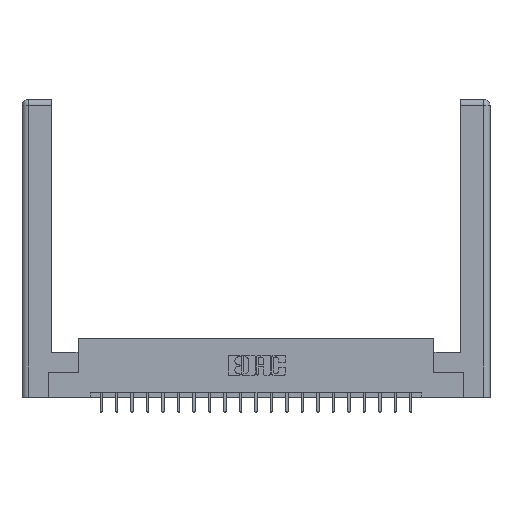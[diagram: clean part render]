
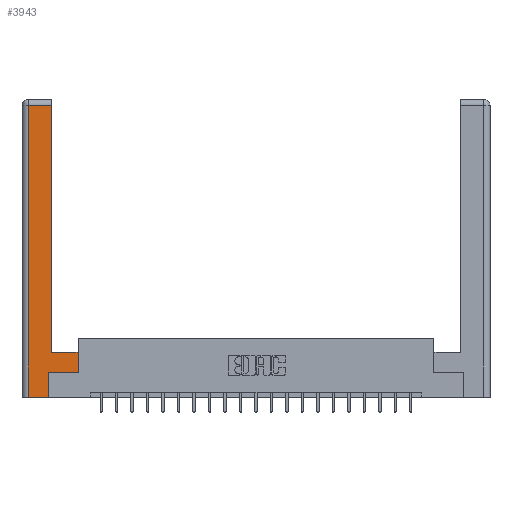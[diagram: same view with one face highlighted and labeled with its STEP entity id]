
A CAD part, top view. The second image highlights one B-rep face of the part: STEP entity #3943.
In plain terms, the highlighted planar face has unit normal (0, 0, 1).
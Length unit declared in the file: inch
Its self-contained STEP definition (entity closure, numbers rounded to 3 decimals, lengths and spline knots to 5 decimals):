
#540 = LINE ( 'NONE', #18890, #16519 ) ;
#795 = DIRECTION ( 'NONE',  ( -1., 0., 0. ) ) ;
#811 = EDGE_LOOP ( 'NONE', ( #6011, #13386, #1071, #17610, #8185, #5318, #9160, #10498 ) ) ;
#840 = VECTOR ( 'NONE', #19273, 39.37008 ) ;
#893 = EDGE_CURVE ( 'NONE', #18559, #1119, #18105, .T. ) ;
#1071 = ORIENTED_EDGE ( 'NONE', *, *, #3435, .T. ) ;
#1119 = VERTEX_POINT ( 'NONE', #12727 ) ;
#1595 = EDGE_CURVE ( 'NONE', #2181, #20528, #540, .T. ) ;
#2181 = VERTEX_POINT ( 'NONE', #11145 ) ;
#2220 = CARTESIAN_POINT ( 'NONE',  ( 0.295, 2.94, 0. ) ) ;
#2565 = EDGE_CURVE ( 'NONE', #6105, #2181, #20928, .T. ) ;
#3435 = EDGE_CURVE ( 'NONE', #1119, #8677, #11996, .T. ) ;
#3753 = CARTESIAN_POINT ( 'NONE',  ( 0.0615, 0., 0. ) ) ;
#3825 = DIRECTION ( 'NONE',  ( -1., 0., 0. ) ) ;
#3943 = ADVANCED_FACE ( 'NONE', ( #18073 ), #9119, .F. ) ;
#5196 = EDGE_CURVE ( 'NONE', #15218, #6105, #16228, .T. ) ;
#5318 = ORIENTED_EDGE ( 'NONE', *, *, #5196, .T. ) ;
#5911 = CARTESIAN_POINT ( 'NONE',  ( 0., 0., 0. ) ) ;
#6011 = ORIENTED_EDGE ( 'NONE', *, *, #12866, .T. ) ;
#6105 = VERTEX_POINT ( 'NONE', #11864 ) ;
#7302 = CARTESIAN_POINT ( 'NONE',  ( 0.0615, 2.94, 0. ) ) ;
#7859 = VECTOR ( 'NONE', #21332, 39.37008 ) ;
#7906 = VERTEX_POINT ( 'NONE', #12146 ) ;
#7962 = EDGE_CURVE ( 'NONE', #7906, #15218, #21311, .T. ) ;
#8045 = VECTOR ( 'NONE', #16902, 39.37008 ) ;
#8185 = ORIENTED_EDGE ( 'NONE', *, *, #7962, .T. ) ;
#8485 = CARTESIAN_POINT ( 'NONE',  ( 0.565, 0.45, 0. ) ) ;
#8677 = VERTEX_POINT ( 'NONE', #3753 ) ;
#9119 = PLANE ( 'NONE',  #15578 ) ;
#9160 = ORIENTED_EDGE ( 'NONE', *, *, #2565, .T. ) ;
#9291 = EDGE_CURVE ( 'NONE', #8677, #7906, #17596, .T. ) ;
#9335 = CARTESIAN_POINT ( 'NONE',  ( 0.295, 0.45, 0. ) ) ;
#9448 = CARTESIAN_POINT ( 'NONE',  ( 0.265, 0., 0. ) ) ;
#10498 = ORIENTED_EDGE ( 'NONE', *, *, #1595, .T. ) ;
#10689 = DIRECTION ( 'NONE',  ( 0., 1., 0. ) ) ;
#10810 = DIRECTION ( 'NONE',  ( -1., 0., 0. ) ) ;
#11069 = DIRECTION ( 'NONE',  ( 1., 0., 0. ) ) ;
#11145 = CARTESIAN_POINT ( 'NONE',  ( 0.565, 0.45, 0. ) ) ;
#11864 = CARTESIAN_POINT ( 'NONE',  ( 0.565, 0.245, 0. ) ) ;
#11996 = LINE ( 'NONE', #15237, #8045 ) ;
#12146 = CARTESIAN_POINT ( 'NONE',  ( 0.265, 0., 0. ) ) ;
#12727 = CARTESIAN_POINT ( 'NONE',  ( 0.0615, 2.94, 0. ) ) ;
#12866 = EDGE_CURVE ( 'NONE', #20528, #18559, #19707, .T. ) ;
#13386 = ORIENTED_EDGE ( 'NONE', *, *, #893, .T. ) ;
#14033 = CARTESIAN_POINT ( 'NONE',  ( 0.295, 3., 0. ) ) ;
#15218 = VERTEX_POINT ( 'NONE', #21317 ) ;
#15237 = CARTESIAN_POINT ( 'NONE',  ( 0.0615, 0., 0. ) ) ;
#15578 = AXIS2_PLACEMENT_3D ( 'NONE', #5911, #15795, #10810 ) ;
#15795 = DIRECTION ( 'NONE',  ( 0., 0., -1. ) ) ;
#16105 = CARTESIAN_POINT ( 'NONE',  ( 0.565, 0.245, 0. ) ) ;
#16228 = LINE ( 'NONE', #16105, #7859 ) ;
#16519 = VECTOR ( 'NONE', #795, 39.37008 ) ;
#16867 = VECTOR ( 'NONE', #10689, 39.37008 ) ;
#16902 = DIRECTION ( 'NONE',  ( 0., -1., 0. ) ) ;
#17069 = VECTOR ( 'NONE', #11069, 39.37008 ) ;
#17275 = CARTESIAN_POINT ( 'NONE',  ( 0.265, 0.245, 0. ) ) ;
#17596 = LINE ( 'NONE', #9448, #17069 ) ;
#17610 = ORIENTED_EDGE ( 'NONE', *, *, #9291, .T. ) ;
#18073 = FACE_OUTER_BOUND ( 'NONE', #811, .T. ) ;
#18105 = LINE ( 'NONE', #7302, #19954 ) ;
#18559 = VERTEX_POINT ( 'NONE', #2220 ) ;
#18890 = CARTESIAN_POINT ( 'NONE',  ( 0.295, 0.45, 0. ) ) ;
#19273 = DIRECTION ( 'NONE',  ( 0., 1., 0. ) ) ;
#19604 = VECTOR ( 'NONE', #20106, 39.37008 ) ;
#19707 = LINE ( 'NONE', #14033, #840 ) ;
#19954 = VECTOR ( 'NONE', #3825, 39.37008 ) ;
#20106 = DIRECTION ( 'NONE',  ( 0., 1., 0. ) ) ;
#20528 = VERTEX_POINT ( 'NONE', #9335 ) ;
#20928 = LINE ( 'NONE', #8485, #19604 ) ;
#21311 = LINE ( 'NONE', #17275, #16867 ) ;
#21317 = CARTESIAN_POINT ( 'NONE',  ( 0.265, 0.245, 0. ) ) ;
#21332 = DIRECTION ( 'NONE',  ( 1., 0., 0. ) ) ;
